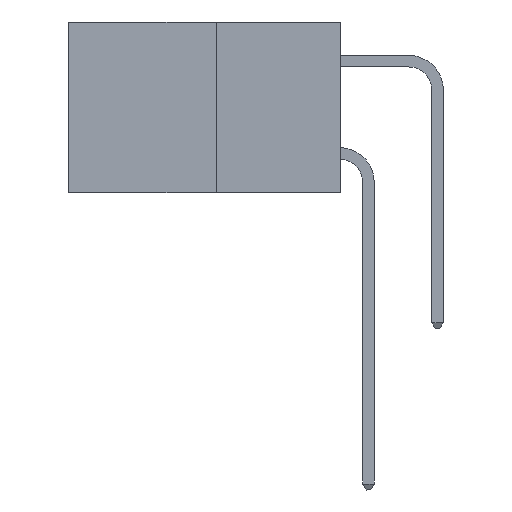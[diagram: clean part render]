
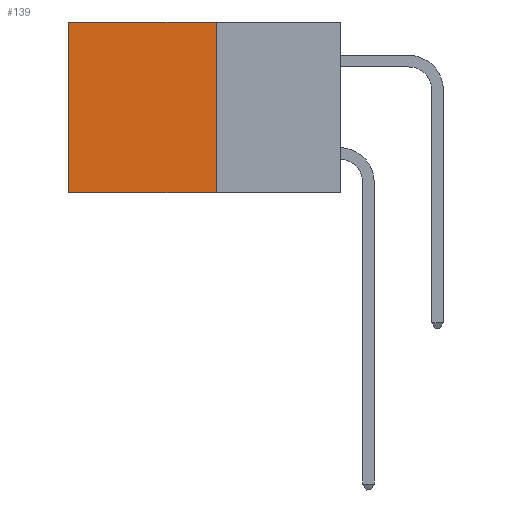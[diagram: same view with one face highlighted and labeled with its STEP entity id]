
A CAD part, left-side view. The second image highlights one B-rep face of the part: STEP entity #139.
In plain terms, the highlighted planar face has unit normal (-1, 0, 0).
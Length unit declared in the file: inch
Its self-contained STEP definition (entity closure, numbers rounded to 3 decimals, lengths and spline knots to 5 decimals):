
#58 = VECTOR ( 'NONE', #7542, 39.37008 ) ;
#139 = ADVANCED_FACE ( 'NONE', ( #1135 ), #238, .F. ) ;
#238 = PLANE ( 'NONE',  #2271 ) ;
#529 = CARTESIAN_POINT ( 'NONE',  ( 0.277, 0.27, 0. ) ) ;
#539 = CARTESIAN_POINT ( 'NONE',  ( 0.277, 0.27, -0.37 ) ) ;
#1135 = FACE_OUTER_BOUND ( 'NONE', #7853, .T. ) ;
#1190 = LINE ( 'NONE', #6524, #8863 ) ;
#1410 = CARTESIAN_POINT ( 'NONE',  ( 0.277, 0.59, -0.37 ) ) ;
#2271 = AXIS2_PLACEMENT_3D ( 'NONE', #3981, #8662, #9531 ) ;
#2280 = LINE ( 'NONE', #539, #9201 ) ;
#2450 = CARTESIAN_POINT ( 'NONE',  ( 0.277, 0.59, 0. ) ) ;
#2455 = EDGE_CURVE ( 'NONE', #8048, #3057, #9631, .T. ) ;
#2956 = ORIENTED_EDGE ( 'NONE', *, *, #8943, .T. ) ;
#3057 = VERTEX_POINT ( 'NONE', #8564 ) ;
#3971 = VECTOR ( 'NONE', #5291, 39.37008 ) ;
#3981 = CARTESIAN_POINT ( 'NONE',  ( 0.277, 0.27, -0.37 ) ) ;
#4082 = LINE ( 'NONE', #5232, #58 ) ;
#4195 = ORIENTED_EDGE ( 'NONE', *, *, #7554, .T. ) ;
#4275 = DIRECTION ( 'NONE',  ( 0., 1., 0. ) ) ;
#4446 = ORIENTED_EDGE ( 'NONE', *, *, #2455, .F. ) ;
#4608 = VERTEX_POINT ( 'NONE', #2450 ) ;
#4873 = VERTEX_POINT ( 'NONE', #1410 ) ;
#5232 = CARTESIAN_POINT ( 'NONE',  ( 0.277, 0.59, -0.37 ) ) ;
#5291 = DIRECTION ( 'NONE',  ( 0., 0., -1. ) ) ;
#6271 = CARTESIAN_POINT ( 'NONE',  ( 0.277, 0.27, -0.37 ) ) ;
#6524 = CARTESIAN_POINT ( 'NONE',  ( 0.277, 0.27, 0. ) ) ;
#7295 = DIRECTION ( 'NONE',  ( 0., 1., 0. ) ) ;
#7418 = EDGE_CURVE ( 'NONE', #3057, #4873, #2280, .T. ) ;
#7542 = DIRECTION ( 'NONE',  ( 0., 0., -1. ) ) ;
#7554 = EDGE_CURVE ( 'NONE', #4608, #4873, #4082, .T. ) ;
#7853 = EDGE_LOOP ( 'NONE', ( #4195, #8230, #4446, #2956 ) ) ;
#8048 = VERTEX_POINT ( 'NONE', #529 ) ;
#8230 = ORIENTED_EDGE ( 'NONE', *, *, #7418, .F. ) ;
#8564 = CARTESIAN_POINT ( 'NONE',  ( 0.277, 0.27, -0.37 ) ) ;
#8662 = DIRECTION ( 'NONE',  ( 1., 0., 0. ) ) ;
#8863 = VECTOR ( 'NONE', #7295, 39.37008 ) ;
#8943 = EDGE_CURVE ( 'NONE', #8048, #4608, #1190, .T. ) ;
#9201 = VECTOR ( 'NONE', #4275, 39.37008 ) ;
#9531 = DIRECTION ( 'NONE',  ( 0., 0., -1. ) ) ;
#9631 = LINE ( 'NONE', #6271, #3971 ) ;
